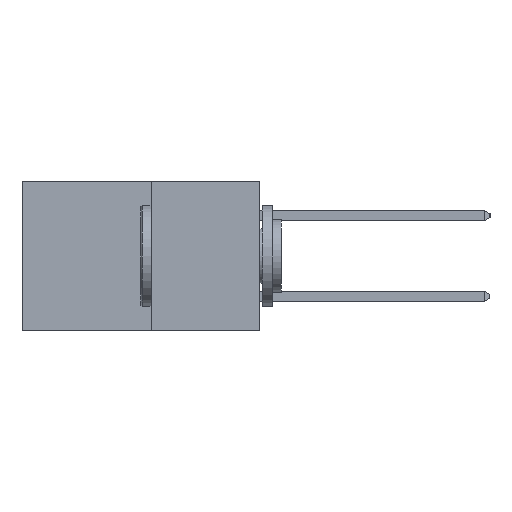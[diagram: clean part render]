
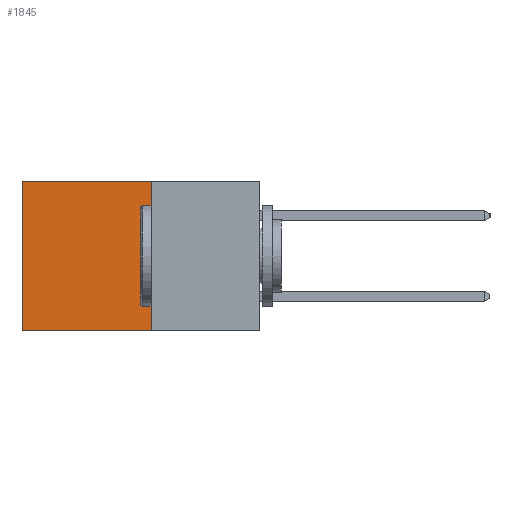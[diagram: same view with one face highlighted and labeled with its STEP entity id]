
A CAD part, left-side view. The second image highlights one B-rep face of the part: STEP entity #1845.
In plain terms, the highlighted planar face has unit normal (-1, 0, 0).
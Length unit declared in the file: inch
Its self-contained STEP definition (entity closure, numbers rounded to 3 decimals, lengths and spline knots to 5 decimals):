
#984 = PLANE ( 'NONE',  #18835 ) ;
#1642 = CARTESIAN_POINT ( 'NONE',  ( 0.277, 0.59, -0.37 ) ) ;
#1845 = ADVANCED_FACE ( 'NONE', ( #26285 ), #984, .F. ) ;
#2517 = LINE ( 'NONE', #22918, #24483 ) ;
#3009 = EDGE_CURVE ( 'NONE', #16291, #26548, #2517, .T. ) ;
#3911 = DIRECTION ( 'NONE',  ( 0., 0., -1. ) ) ;
#4508 = DIRECTION ( 'NONE',  ( 0., 1., 0. ) ) ;
#5785 = CARTESIAN_POINT ( 'NONE',  ( 0.277, 0.59, -0.37 ) ) ;
#6650 = ORIENTED_EDGE ( 'NONE', *, *, #13702, .F. ) ;
#7035 = EDGE_CURVE ( 'NONE', #16291, #10467, #23641, .T. ) ;
#8085 = ORIENTED_EDGE ( 'NONE', *, *, #14623, .T. ) ;
#9320 = ORIENTED_EDGE ( 'NONE', *, *, #7035, .T. ) ;
#9357 = ORIENTED_EDGE ( 'NONE', *, *, #3009, .F. ) ;
#9760 = CARTESIAN_POINT ( 'NONE',  ( 0.277, 0.59, 0. ) ) ;
#10467 = VERTEX_POINT ( 'NONE', #9760 ) ;
#10875 = EDGE_LOOP ( 'NONE', ( #8085, #6650, #9357, #9320 ) ) ;
#11636 = DIRECTION ( 'NONE',  ( 0., 0., -1. ) ) ;
#13311 = CARTESIAN_POINT ( 'NONE',  ( 0.277, 0.27, 0. ) ) ;
#13702 = EDGE_CURVE ( 'NONE', #26548, #22728, #21548, .T. ) ;
#14623 = EDGE_CURVE ( 'NONE', #10467, #22728, #15531, .T. ) ;
#14816 = VECTOR ( 'NONE', #3911, 39.37008 ) ;
#15531 = LINE ( 'NONE', #1642, #14816 ) ;
#15876 = CARTESIAN_POINT ( 'NONE',  ( 0.277, 0.27, -0.37 ) ) ;
#16291 = VERTEX_POINT ( 'NONE', #25101 ) ;
#18422 = VECTOR ( 'NONE', #28889, 39.37008 ) ;
#18835 = AXIS2_PLACEMENT_3D ( 'NONE', #26908, #27590, #11636 ) ;
#20530 = DIRECTION ( 'NONE',  ( 0., 0., -1. ) ) ;
#21548 = LINE ( 'NONE', #15876, #26770 ) ;
#22728 = VERTEX_POINT ( 'NONE', #5785 ) ;
#22918 = CARTESIAN_POINT ( 'NONE',  ( 0.277, 0.27, -0.37 ) ) ;
#23641 = LINE ( 'NONE', #13311, #18422 ) ;
#24483 = VECTOR ( 'NONE', #20530, 39.37008 ) ;
#25101 = CARTESIAN_POINT ( 'NONE',  ( 0.277, 0.27, 0. ) ) ;
#26285 = FACE_OUTER_BOUND ( 'NONE', #10875, .T. ) ;
#26548 = VERTEX_POINT ( 'NONE', #28273 ) ;
#26770 = VECTOR ( 'NONE', #4508, 39.37008 ) ;
#26908 = CARTESIAN_POINT ( 'NONE',  ( 0.277, 0.27, -0.37 ) ) ;
#27590 = DIRECTION ( 'NONE',  ( 1., 0., 0. ) ) ;
#28273 = CARTESIAN_POINT ( 'NONE',  ( 0.277, 0.27, -0.37 ) ) ;
#28889 = DIRECTION ( 'NONE',  ( 0., 1., 0. ) ) ;
